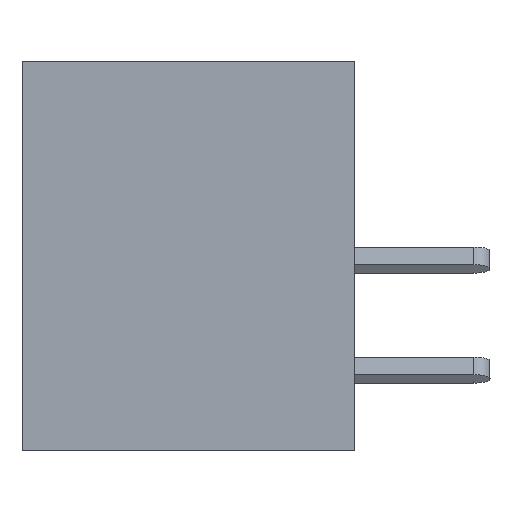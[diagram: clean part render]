
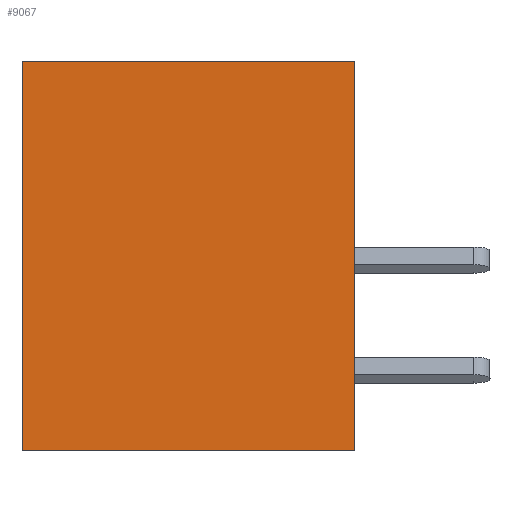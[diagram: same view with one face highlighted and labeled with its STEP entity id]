
A CAD part, left-side view. The second image highlights one B-rep face of the part: STEP entity #9067.
In plain terms, the highlighted planar face has unit normal (-1, 0, 0).
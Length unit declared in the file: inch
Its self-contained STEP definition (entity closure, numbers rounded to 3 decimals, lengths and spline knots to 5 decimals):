
#158 = CARTESIAN_POINT ( 'NONE',  ( 0., 0.453, 0. ) ) ;
#441 = VERTEX_POINT ( 'NONE', #17176 ) ;
#1086 = ORIENTED_EDGE ( 'NONE', *, *, #4513, .F. ) ;
#1596 = PLANE ( 'NONE',  #20226 ) ;
#1942 = DIRECTION ( 'NONE',  ( 0., -1., 0. ) ) ;
#2921 = CARTESIAN_POINT ( 'NONE',  ( 0., 0.453, -0.531 ) ) ;
#4305 = LINE ( 'NONE', #16473, #16068 ) ;
#4513 = EDGE_CURVE ( 'NONE', #10129, #8463, #7159, .T. ) ;
#4690 = VERTEX_POINT ( 'NONE', #16599 ) ;
#4902 = DIRECTION ( 'NONE',  ( 1., 0., 0. ) ) ;
#5298 = DIRECTION ( 'NONE',  ( 0., 0., 1. ) ) ;
#5364 = EDGE_CURVE ( 'NONE', #441, #4690, #20358, .T. ) ;
#5998 = DIRECTION ( 'NONE',  ( 0., -1., 0. ) ) ;
#7159 = LINE ( 'NONE', #158, #20611 ) ;
#7380 = DIRECTION ( 'NONE',  ( 0., 0., 1. ) ) ;
#7472 = EDGE_CURVE ( 'NONE', #4690, #8463, #16444, .T. ) ;
#8463 = VERTEX_POINT ( 'NONE', #17789 ) ;
#8478 = EDGE_LOOP ( 'NONE', ( #15311, #1086, #10887, #9864 ) ) ;
#9067 = ADVANCED_FACE ( 'NONE', ( #11384 ), #1596, .F. ) ;
#9151 = VECTOR ( 'NONE', #5998, 39.37008 ) ;
#9864 = ORIENTED_EDGE ( 'NONE', *, *, #5364, .T. ) ;
#10129 = VERTEX_POINT ( 'NONE', #18903 ) ;
#10465 = VECTOR ( 'NONE', #7380, 39.37008 ) ;
#10887 = ORIENTED_EDGE ( 'NONE', *, *, #16336, .F. ) ;
#11284 = DIRECTION ( 'NONE',  ( 0., 0., -1. ) ) ;
#11384 = FACE_OUTER_BOUND ( 'NONE', #8478, .T. ) ;
#14091 = CARTESIAN_POINT ( 'NONE',  ( 0., 0., 0. ) ) ;
#15311 = ORIENTED_EDGE ( 'NONE', *, *, #7472, .T. ) ;
#15956 = CARTESIAN_POINT ( 'NONE',  ( 0., 0.453, 0. ) ) ;
#16068 = VECTOR ( 'NONE', #5298, 39.37008 ) ;
#16336 = EDGE_CURVE ( 'NONE', #441, #10129, #4305, .T. ) ;
#16444 = LINE ( 'NONE', #14091, #10465 ) ;
#16473 = CARTESIAN_POINT ( 'NONE',  ( 0., 0.453, 0. ) ) ;
#16599 = CARTESIAN_POINT ( 'NONE',  ( 0., 0., -0.531 ) ) ;
#17176 = CARTESIAN_POINT ( 'NONE',  ( 0., 0.453, -0.531 ) ) ;
#17789 = CARTESIAN_POINT ( 'NONE',  ( 0., 0., 0. ) ) ;
#18903 = CARTESIAN_POINT ( 'NONE',  ( 0., 0.453, 0. ) ) ;
#20226 = AXIS2_PLACEMENT_3D ( 'NONE', #15956, #4902, #11284 ) ;
#20358 = LINE ( 'NONE', #2921, #9151 ) ;
#20611 = VECTOR ( 'NONE', #1942, 39.37008 ) ;
